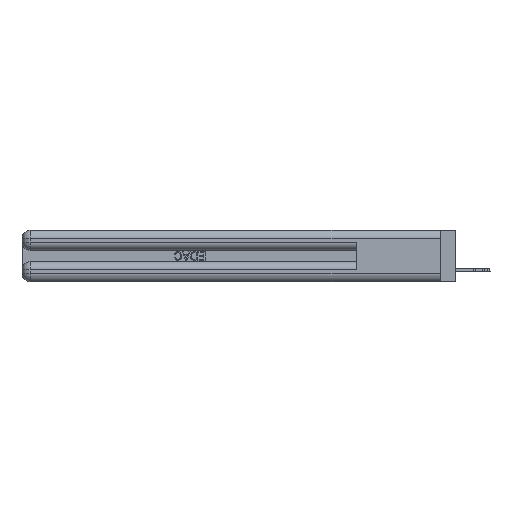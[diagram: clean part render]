
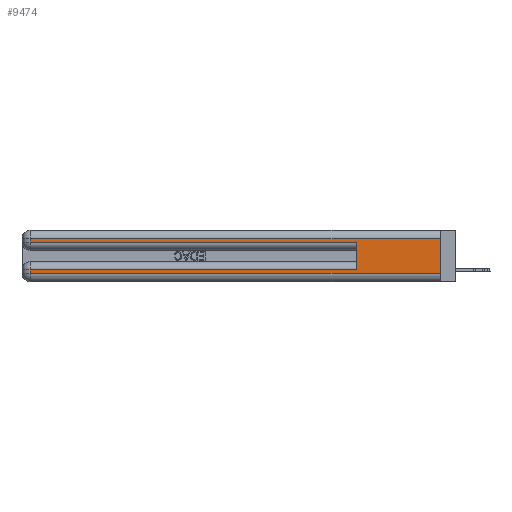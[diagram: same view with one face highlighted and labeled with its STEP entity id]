
A CAD part, left-side view. The second image highlights one B-rep face of the part: STEP entity #9474.
In plain terms, the highlighted planar face has unit normal (-1, 0, 0).
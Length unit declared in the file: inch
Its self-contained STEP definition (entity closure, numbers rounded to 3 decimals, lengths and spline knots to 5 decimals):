
#274 = FACE_OUTER_BOUND ( 'NONE', #3541, .T. ) ;
#483 = VERTEX_POINT ( 'NONE', #21319 ) ;
#513 = ORIENTED_EDGE ( 'NONE', *, *, #31818, .T. ) ;
#946 = LINE ( 'NONE', #28526, #29965 ) ;
#1183 = VECTOR ( 'NONE', #20046, 39.37008 ) ;
#1596 = DIRECTION ( 'NONE',  ( 0., 0., -1. ) ) ;
#3541 = EDGE_LOOP ( 'NONE', ( #34591, #15610, #11329, #17618, #26879, #16310, #24520, #513 ) ) ;
#4163 = VERTEX_POINT ( 'NONE', #10772 ) ;
#6111 = VERTEX_POINT ( 'NONE', #50543 ) ;
#9068 = EDGE_CURVE ( 'NONE', #14397, #483, #35382, .T. ) ;
#9474 = ADVANCED_FACE ( 'NONE', ( #274 ), #17936, .F. ) ;
#9970 = CARTESIAN_POINT ( 'NONE',  ( 0., 0.6, 0.285 ) ) ;
#10772 = CARTESIAN_POINT ( 'NONE',  ( 0., 0., 0.06 ) ) ;
#11329 = ORIENTED_EDGE ( 'NONE', *, *, #34038, .T. ) ;
#12006 = EDGE_CURVE ( 'NONE', #30122, #49554, #47784, .T. ) ;
#12065 = LINE ( 'NONE', #12083, #37825 ) ;
#12083 = CARTESIAN_POINT ( 'NONE',  ( 0., 0., 0.06 ) ) ;
#12609 = CARTESIAN_POINT ( 'NONE',  ( 0., 2.94, 0.06 ) ) ;
#14397 = VERTEX_POINT ( 'NONE', #21505 ) ;
#15610 = ORIENTED_EDGE ( 'NONE', *, *, #49865, .T. ) ;
#16310 = ORIENTED_EDGE ( 'NONE', *, *, #9068, .T. ) ;
#16378 = CARTESIAN_POINT ( 'NONE',  ( 0., 0.6, 0.145 ) ) ;
#16771 = DIRECTION ( 'NONE',  ( 0., -1., 0. ) ) ;
#17618 = ORIENTED_EDGE ( 'NONE', *, *, #12006, .T. ) ;
#17936 = PLANE ( 'NONE',  #34731 ) ;
#20046 = DIRECTION ( 'NONE',  ( 0., 0., 1. ) ) ;
#21319 = CARTESIAN_POINT ( 'NONE',  ( 0., 2.94, 0.085 ) ) ;
#21505 = CARTESIAN_POINT ( 'NONE',  ( 0., 0.6, 0.085 ) ) ;
#22971 = DIRECTION ( 'NONE',  ( 0., 1., 0. ) ) ;
#23885 = CARTESIAN_POINT ( 'NONE',  ( 0., 2.94, 0.37 ) ) ;
#24520 = ORIENTED_EDGE ( 'NONE', *, *, #44948, .T. ) ;
#24622 = DIRECTION ( 'NONE',  ( 0., 0., -1. ) ) ;
#25041 = CARTESIAN_POINT ( 'NONE',  ( 0., 0., 0.285 ) ) ;
#26738 = CARTESIAN_POINT ( 'NONE',  ( 0., 0., 0.37 ) ) ;
#26879 = ORIENTED_EDGE ( 'NONE', *, *, #36417, .F. ) ;
#27477 = VECTOR ( 'NONE', #36378, 39.37008 ) ;
#28526 = CARTESIAN_POINT ( 'NONE',  ( 0., 0., 0.37 ) ) ;
#28768 = DIRECTION ( 'NONE',  ( 0., -1., 0. ) ) ;
#29947 = LINE ( 'NONE', #23885, #27477 ) ;
#29965 = VECTOR ( 'NONE', #24622, 39.37008 ) ;
#30122 = VERTEX_POINT ( 'NONE', #52059 ) ;
#30996 = DIRECTION ( 'NONE',  ( 1., 0., 0. ) ) ;
#31233 = CARTESIAN_POINT ( 'NONE',  ( 0., 2.94, 0.31 ) ) ;
#31818 = EDGE_CURVE ( 'NONE', #34250, #4163, #12065, .T. ) ;
#34038 = EDGE_CURVE ( 'NONE', #51665, #30122, #29947, .T. ) ;
#34250 = VERTEX_POINT ( 'NONE', #12609 ) ;
#34591 = ORIENTED_EDGE ( 'NONE', *, *, #51797, .F. ) ;
#34731 = AXIS2_PLACEMENT_3D ( 'NONE', #26738, #30996, #42464 ) ;
#35382 = LINE ( 'NONE', #51446, #44864 ) ;
#36378 = DIRECTION ( 'NONE',  ( 0., 0., -1. ) ) ;
#36417 = EDGE_CURVE ( 'NONE', #14397, #49554, #38454, .T. ) ;
#36990 = VECTOR ( 'NONE', #1596, 39.37008 ) ;
#37825 = VECTOR ( 'NONE', #16771, 39.37008 ) ;
#38454 = LINE ( 'NONE', #16378, #1183 ) ;
#38834 = VECTOR ( 'NONE', #28768, 39.37008 ) ;
#41516 = LINE ( 'NONE', #47937, #42178 ) ;
#42066 = LINE ( 'NONE', #49959, #36990 ) ;
#42178 = VECTOR ( 'NONE', #44001, 39.37008 ) ;
#42464 = DIRECTION ( 'NONE',  ( 0., 0., -1. ) ) ;
#44001 = DIRECTION ( 'NONE',  ( 0., 1., 0. ) ) ;
#44864 = VECTOR ( 'NONE', #22971, 39.37008 ) ;
#44948 = EDGE_CURVE ( 'NONE', #483, #34250, #42066, .T. ) ;
#47784 = LINE ( 'NONE', #25041, #38834 ) ;
#47937 = CARTESIAN_POINT ( 'NONE',  ( 0., 0., 0.31 ) ) ;
#49554 = VERTEX_POINT ( 'NONE', #9970 ) ;
#49865 = EDGE_CURVE ( 'NONE', #6111, #51665, #41516, .T. ) ;
#49959 = CARTESIAN_POINT ( 'NONE',  ( 0., 2.94, 0.37 ) ) ;
#50543 = CARTESIAN_POINT ( 'NONE',  ( 0., 0., 0.31 ) ) ;
#51446 = CARTESIAN_POINT ( 'NONE',  ( 0., 0., 0.085 ) ) ;
#51665 = VERTEX_POINT ( 'NONE', #31233 ) ;
#51797 = EDGE_CURVE ( 'NONE', #6111, #4163, #946, .T. ) ;
#52059 = CARTESIAN_POINT ( 'NONE',  ( 0., 2.94, 0.285 ) ) ;
